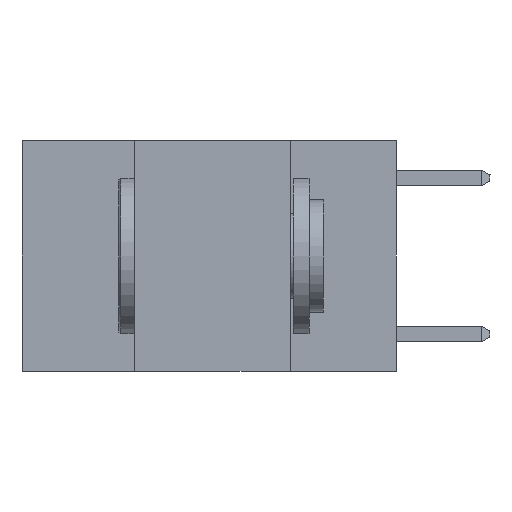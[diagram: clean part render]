
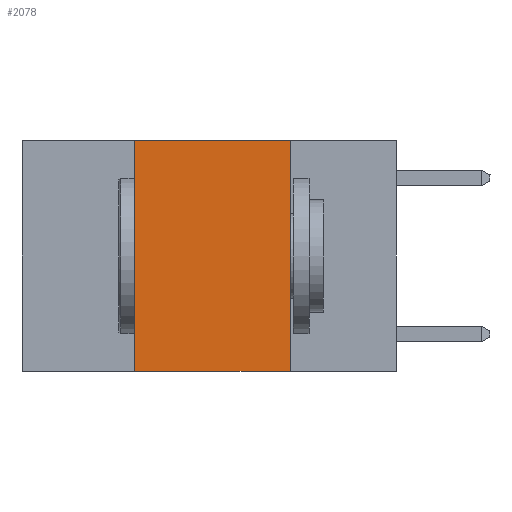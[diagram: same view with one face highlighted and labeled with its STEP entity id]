
A CAD part, left-side view. The second image highlights one B-rep face of the part: STEP entity #2078.
In plain terms, the highlighted planar face has unit normal (-1, 0, 0).
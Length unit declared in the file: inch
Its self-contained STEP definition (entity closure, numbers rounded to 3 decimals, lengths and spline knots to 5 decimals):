
#71 = DIRECTION ( 'NONE',  ( 0., 0., -1. ) ) ;
#957 = CARTESIAN_POINT ( 'NONE',  ( 0., 0.6, -0.37 ) ) ;
#1372 = VERTEX_POINT ( 'NONE', #4337 ) ;
#2076 = ORIENTED_EDGE ( 'NONE', *, *, #11137, .F. ) ;
#2078 = ADVANCED_FACE ( 'NONE', ( #14206 ), #4155, .F. ) ;
#2292 = ORIENTED_EDGE ( 'NONE', *, *, #6236, .F. ) ;
#2388 = LINE ( 'NONE', #957, #13501 ) ;
#2517 = CARTESIAN_POINT ( 'NONE',  ( 0., 0.17, 0. ) ) ;
#3453 = VECTOR ( 'NONE', #6405, 39.37008 ) ;
#4155 = PLANE ( 'NONE',  #6773 ) ;
#4337 = CARTESIAN_POINT ( 'NONE',  ( 0., 0.42, -0.37 ) ) ;
#4733 = EDGE_CURVE ( 'NONE', #1372, #6825, #2388, .T. ) ;
#5029 = CARTESIAN_POINT ( 'NONE',  ( 0., 0.42, 0. ) ) ;
#6236 = EDGE_CURVE ( 'NONE', #1372, #10956, #11215, .T. ) ;
#6405 = DIRECTION ( 'NONE',  ( 0., -1., 0. ) ) ;
#6436 = DIRECTION ( 'NONE',  ( 0., 0., -1. ) ) ;
#6464 = LINE ( 'NONE', #7456, #3453 ) ;
#6560 = VECTOR ( 'NONE', #12754, 39.37008 ) ;
#6773 = AXIS2_PLACEMENT_3D ( 'NONE', #11690, #12726, #6436 ) ;
#6825 = VERTEX_POINT ( 'NONE', #10469 ) ;
#7456 = CARTESIAN_POINT ( 'NONE',  ( 0., 0.6, 0. ) ) ;
#7528 = CARTESIAN_POINT ( 'NONE',  ( 0., 0.42, 0. ) ) ;
#8458 = VECTOR ( 'NONE', #71, 39.37008 ) ;
#9135 = EDGE_LOOP ( 'NONE', ( #10445, #2076, #2292, #11635 ) ) ;
#10445 = ORIENTED_EDGE ( 'NONE', *, *, #12583, .F. ) ;
#10469 = CARTESIAN_POINT ( 'NONE',  ( 0., 0.17, -0.37 ) ) ;
#10847 = CARTESIAN_POINT ( 'NONE',  ( 0., 0.17, 0. ) ) ;
#10956 = VERTEX_POINT ( 'NONE', #5029 ) ;
#11137 = EDGE_CURVE ( 'NONE', #10956, #13607, #6464, .T. ) ;
#11215 = LINE ( 'NONE', #7528, #6560 ) ;
#11272 = LINE ( 'NONE', #2517, #8458 ) ;
#11635 = ORIENTED_EDGE ( 'NONE', *, *, #4733, .T. ) ;
#11690 = CARTESIAN_POINT ( 'NONE',  ( 0., 0.6, 0. ) ) ;
#11985 = DIRECTION ( 'NONE',  ( 0., -1., 0. ) ) ;
#12583 = EDGE_CURVE ( 'NONE', #13607, #6825, #11272, .T. ) ;
#12726 = DIRECTION ( 'NONE',  ( 1., 0., 0. ) ) ;
#12754 = DIRECTION ( 'NONE',  ( 0., 0., 1. ) ) ;
#13501 = VECTOR ( 'NONE', #11985, 39.37008 ) ;
#13607 = VERTEX_POINT ( 'NONE', #10847 ) ;
#14206 = FACE_OUTER_BOUND ( 'NONE', #9135, .T. ) ;
